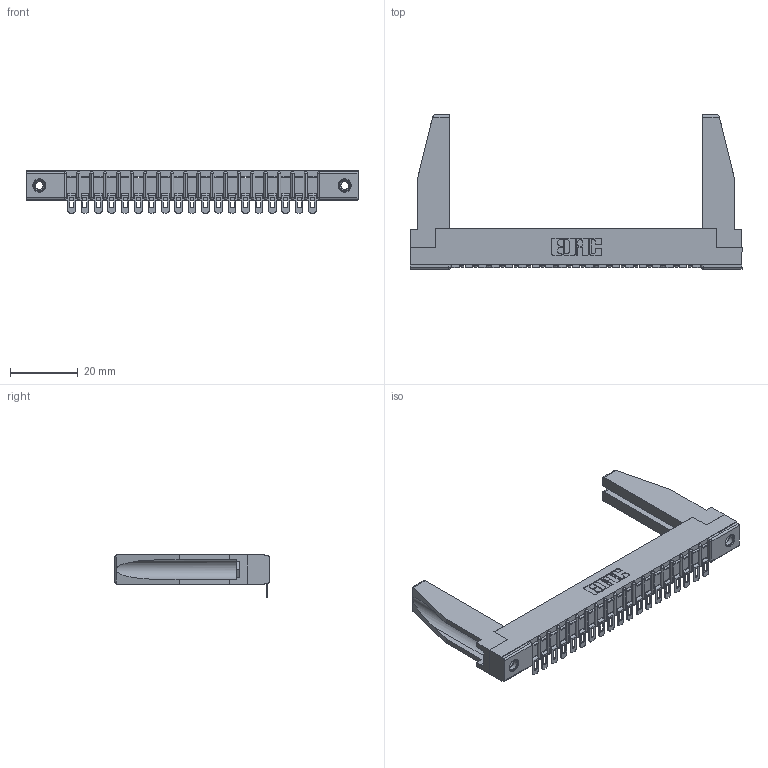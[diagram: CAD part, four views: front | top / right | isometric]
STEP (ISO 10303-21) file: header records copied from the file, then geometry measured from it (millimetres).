
FILE_DESCRIPTION (( 'STEP AP203' ), '1' );
FILE_NAME ('357-019-554-178.STEP', '2019-09-16T22:05:11', ( '' ), ( '' ), 'SwSTEP 2.0', 'SolidWorks 2016', '' );
FILE_SCHEMA (( 'CONFIG_CONTROL_DESIGN' ));
Length unit declared in the file: inch
Products named in the file (5): 307 Part_.156 Dia Mounting Holes; 307-290-002_554; 307-220-078; 345-250-001_345-250-001-102; 357-019-554-178
Assembly tree (24 placements, depth 2):
  357-019-554-178
    307 Part_.156 Dia Mounting Holes
    307-290-002_554  x19
    307-220-078  x2
    345-250-001_345-250-001-102  x2
Bounding box: 98.3 x 45.72 x 12.52 mm (x, y, z)
Volume: 10488 mm3; surface area: 15544.9 mm2
Topology: 24 solids, 24 shells, 1807 faces, 5460 edges, 3576 vertices
Faces by surface type: plane 1028, cylinder 723, sphere 40, cone 12, torus 4
Entity records: 22528 total; most frequent: CARTESIAN_POINT 3796, ORIENTED_EDGE 3742, DIRECTION 3661, EDGE_CURVE 1871, LINE 1419, VECTOR 1419, VERTEX_POINT 1214, AXIS2_PLACEMENT_3D 1121
